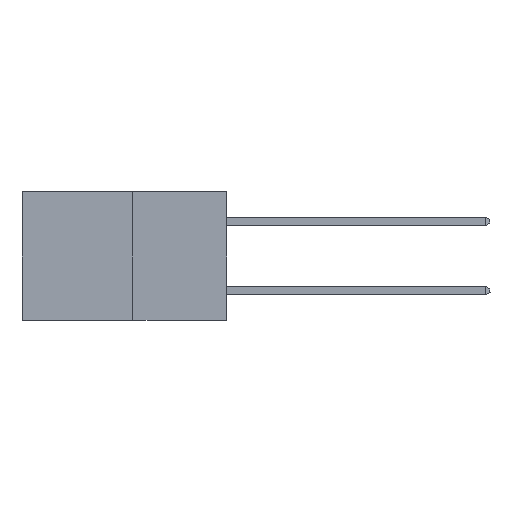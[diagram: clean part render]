
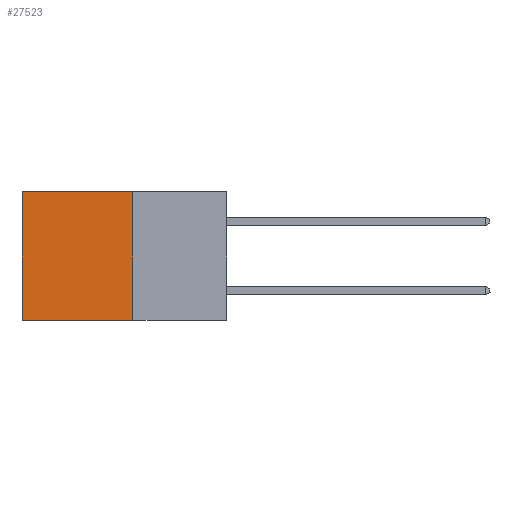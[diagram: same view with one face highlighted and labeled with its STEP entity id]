
A CAD part, left-side view. The second image highlights one B-rep face of the part: STEP entity #27523.
In plain terms, the highlighted planar face has unit normal (-1, 0, 0).
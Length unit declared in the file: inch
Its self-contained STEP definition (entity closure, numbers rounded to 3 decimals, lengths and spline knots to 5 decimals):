
#1804 = LINE ( 'NONE', #17618, #15314 ) ;
#2278 = ORIENTED_EDGE ( 'NONE', *, *, #18376, .T. ) ;
#4496 = CARTESIAN_POINT ( 'NONE',  ( 0.277, 0.27, 0. ) ) ;
#5293 = EDGE_LOOP ( 'NONE', ( #2278, #7081, #8487, #7995 ) ) ;
#6208 = VERTEX_POINT ( 'NONE', #9265 ) ;
#7081 = ORIENTED_EDGE ( 'NONE', *, *, #32666, .F. ) ;
#7244 = DIRECTION ( 'NONE',  ( 0., 1., 0. ) ) ;
#7995 = ORIENTED_EDGE ( 'NONE', *, *, #26290, .T. ) ;
#8487 = ORIENTED_EDGE ( 'NONE', *, *, #32579, .F. ) ;
#9265 = CARTESIAN_POINT ( 'NONE',  ( 0.277, 0.59, 0. ) ) ;
#9805 = PLANE ( 'NONE',  #19438 ) ;
#11169 = VECTOR ( 'NONE', #29458, 39.37008 ) ;
#11995 = VERTEX_POINT ( 'NONE', #20570 ) ;
#12466 = CARTESIAN_POINT ( 'NONE',  ( 0.277, 0.27, -0.37 ) ) ;
#15314 = VECTOR ( 'NONE', #25707, 39.37008 ) ;
#15446 = CARTESIAN_POINT ( 'NONE',  ( 0.277, 0.59, -0.37 ) ) ;
#15759 = LINE ( 'NONE', #19061, #29145 ) ;
#17618 = CARTESIAN_POINT ( 'NONE',  ( 0.277, 0.59, -0.37 ) ) ;
#17862 = DIRECTION ( 'NONE',  ( 0., 0., -1. ) ) ;
#18376 = EDGE_CURVE ( 'NONE', #6208, #20095, #1804, .T. ) ;
#19061 = CARTESIAN_POINT ( 'NONE',  ( 0.277, 0.27, -0.37 ) ) ;
#19438 = AXIS2_PLACEMENT_3D ( 'NONE', #12466, #33875, #17862 ) ;
#19915 = CARTESIAN_POINT ( 'NONE',  ( 0.277, 0.27, 0. ) ) ;
#20095 = VERTEX_POINT ( 'NONE', #15446 ) ;
#20265 = LINE ( 'NONE', #4496, #33653 ) ;
#20570 = CARTESIAN_POINT ( 'NONE',  ( 0.277, 0.27, -0.37 ) ) ;
#24456 = DIRECTION ( 'NONE',  ( 0., 1., 0. ) ) ;
#25707 = DIRECTION ( 'NONE',  ( 0., 0., -1. ) ) ;
#26290 = EDGE_CURVE ( 'NONE', #26668, #6208, #20265, .T. ) ;
#26668 = VERTEX_POINT ( 'NONE', #19915 ) ;
#26796 = CARTESIAN_POINT ( 'NONE',  ( 0.277, 0.27, -0.37 ) ) ;
#27523 = ADVANCED_FACE ( 'NONE', ( #29779 ), #9805, .F. ) ;
#29145 = VECTOR ( 'NONE', #24456, 39.37008 ) ;
#29458 = DIRECTION ( 'NONE',  ( 0., 0., -1. ) ) ;
#29779 = FACE_OUTER_BOUND ( 'NONE', #5293, .T. ) ;
#32520 = LINE ( 'NONE', #26796, #11169 ) ;
#32579 = EDGE_CURVE ( 'NONE', #26668, #11995, #32520, .T. ) ;
#32666 = EDGE_CURVE ( 'NONE', #11995, #20095, #15759, .T. ) ;
#33653 = VECTOR ( 'NONE', #7244, 39.37008 ) ;
#33875 = DIRECTION ( 'NONE',  ( 1., 0., 0. ) ) ;
